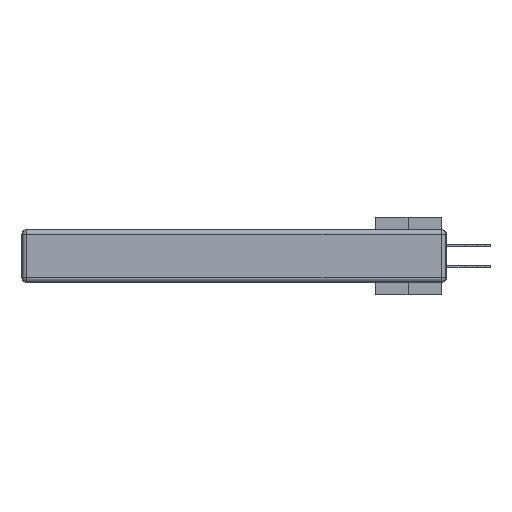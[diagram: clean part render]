
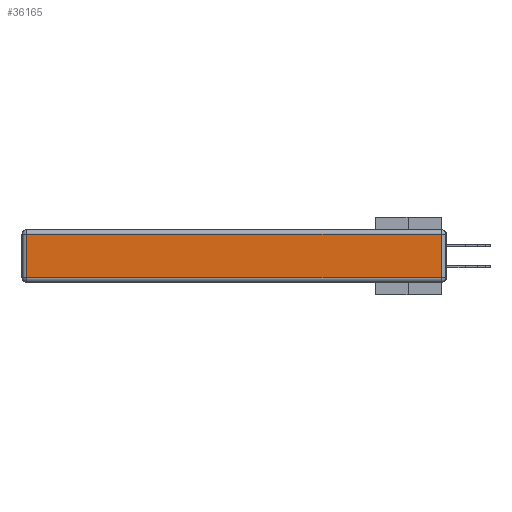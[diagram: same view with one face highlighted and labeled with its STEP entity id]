
A CAD part, left-side view. The second image highlights one B-rep face of the part: STEP entity #36165.
In plain terms, the highlighted planar face has unit normal (-1, 0, 0).
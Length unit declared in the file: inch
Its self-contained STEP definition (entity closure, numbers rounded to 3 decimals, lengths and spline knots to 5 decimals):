
#1023 = ORIENTED_EDGE ( 'NONE', *, *, #7711, .T. ) ;
#1748 = ORIENTED_EDGE ( 'NONE', *, *, #24984, .T. ) ;
#4401 = PLANE ( 'NONE',  #44302 ) ;
#4777 = CARTESIAN_POINT ( 'NONE',  ( 0., 2.72, -0.313 ) ) ;
#7711 = EDGE_CURVE ( 'NONE', #35283, #18245, #38644, .T. ) ;
#8238 = DIRECTION ( 'NONE',  ( 0., 0., 1. ) ) ;
#9578 = VECTOR ( 'NONE', #37444, 39.37008 ) ;
#10722 = LINE ( 'NONE', #39823, #34516 ) ;
#14276 = CARTESIAN_POINT ( 'NONE',  ( 0., 2.75, -0.03 ) ) ;
#15618 = DIRECTION ( 'NONE',  ( -1., 0., 0. ) ) ;
#17250 = VECTOR ( 'NONE', #21937, 39.37008 ) ;
#18138 = ORIENTED_EDGE ( 'NONE', *, *, #43217, .T. ) ;
#18245 = VERTEX_POINT ( 'NONE', #40050 ) ;
#19167 = DIRECTION ( 'NONE',  ( 0., -1., 0. ) ) ;
#21937 = DIRECTION ( 'NONE',  ( 0., 1., 0. ) ) ;
#24407 = LINE ( 'NONE', #45288, #9578 ) ;
#24926 = ORIENTED_EDGE ( 'NONE', *, *, #43419, .T. ) ;
#24984 = EDGE_CURVE ( 'NONE', #25039, #40880, #25237, .T. ) ;
#25039 = VERTEX_POINT ( 'NONE', #4777 ) ;
#25237 = LINE ( 'NONE', #41765, #26410 ) ;
#26410 = VECTOR ( 'NONE', #19167, 39.37008 ) ;
#34364 = FACE_OUTER_BOUND ( 'NONE', #48449, .T. ) ;
#34516 = VECTOR ( 'NONE', #43508, 39.37008 ) ;
#34612 = CARTESIAN_POINT ( 'NONE',  ( 0., 0., -0.343 ) ) ;
#35283 = VERTEX_POINT ( 'NONE', #45270 ) ;
#36165 = ADVANCED_FACE ( 'NONE', ( #34364 ), #4401, .T. ) ;
#37444 = DIRECTION ( 'NONE',  ( 0., 0., -1. ) ) ;
#38644 = LINE ( 'NONE', #14276, #17250 ) ;
#39823 = CARTESIAN_POINT ( 'NONE',  ( 0., 0.03, -0.343 ) ) ;
#40050 = CARTESIAN_POINT ( 'NONE',  ( 0., 2.72, -0.03 ) ) ;
#40880 = VERTEX_POINT ( 'NONE', #47061 ) ;
#41765 = CARTESIAN_POINT ( 'NONE',  ( 0., 0., -0.313 ) ) ;
#43217 = EDGE_CURVE ( 'NONE', #40880, #35283, #10722, .T. ) ;
#43419 = EDGE_CURVE ( 'NONE', #18245, #25039, #24407, .T. ) ;
#43508 = DIRECTION ( 'NONE',  ( 0., 0., 1. ) ) ;
#44302 = AXIS2_PLACEMENT_3D ( 'NONE', #34612, #15618, #8238 ) ;
#45270 = CARTESIAN_POINT ( 'NONE',  ( 0., 0.03, -0.03 ) ) ;
#45288 = CARTESIAN_POINT ( 'NONE',  ( 0., 2.72, -0.343 ) ) ;
#47061 = CARTESIAN_POINT ( 'NONE',  ( 0., 0.03, -0.313 ) ) ;
#48449 = EDGE_LOOP ( 'NONE', ( #1748, #18138, #1023, #24926 ) ) ;
